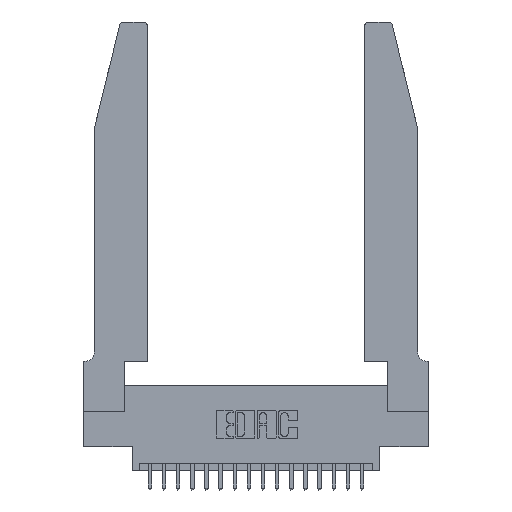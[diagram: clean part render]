
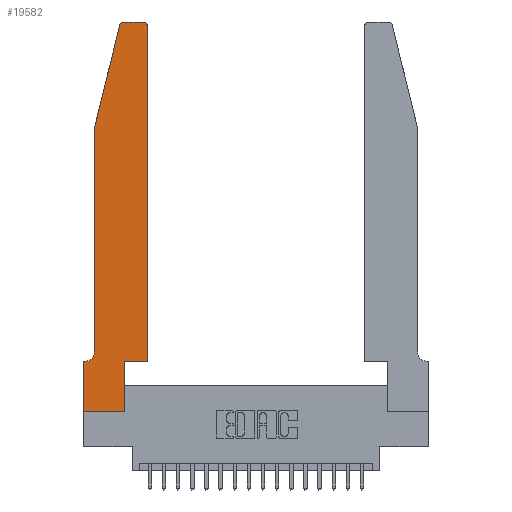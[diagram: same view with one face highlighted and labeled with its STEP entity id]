
A CAD part, top view. The second image highlights one B-rep face of the part: STEP entity #19582.
In plain terms, the highlighted planar face has unit normal (0, 0, 1).
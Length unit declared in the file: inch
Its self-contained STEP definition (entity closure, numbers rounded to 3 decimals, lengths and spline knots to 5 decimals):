
#254 = CARTESIAN_POINT ( 'NONE',  ( 0.284, 2.72, 0.37 ) ) ;
#951 = EDGE_CURVE ( 'NONE', #15937, #16300, #12859, .T. ) ;
#1006 = VECTOR ( 'NONE', #16605, 39.37008 ) ;
#1920 = DIRECTION ( 'NONE',  ( 1., 0., 0. ) ) ;
#2243 = DIRECTION ( 'NONE',  ( 1., 0., 0. ) ) ;
#2263 = DIRECTION ( 'NONE',  ( 0., -1., 0. ) ) ;
#2414 = CARTESIAN_POINT ( 'NONE',  ( 0.4505, 0.35, 0.37 ) ) ;
#2462 = AXIS2_PLACEMENT_3D ( 'NONE', #9219, #19206, #9296 ) ;
#2728 = CARTESIAN_POINT ( 'NONE',  ( 0., 0., 0.37 ) ) ;
#2730 = CIRCLE ( 'NONE', #2462, 0.03 ) ;
#2776 = VECTOR ( 'NONE', #20815, 39.37008 ) ;
#2783 = ORIENTED_EDGE ( 'NONE', *, *, #6001, .T. ) ;
#3015 = EDGE_CURVE ( 'NONE', #16300, #16462, #18865, .T. ) ;
#3296 = ORIENTED_EDGE ( 'NONE', *, *, #18633, .T. ) ;
#3348 = VERTEX_POINT ( 'NONE', #7384 ) ;
#3589 = CARTESIAN_POINT ( 'NONE',  ( 0.4505, 0.35, 0.37 ) ) ;
#3684 = CARTESIAN_POINT ( 'NONE',  ( 0.2605, 2.75, 0.37 ) ) ;
#3708 = EDGE_CURVE ( 'NONE', #10830, #5366, #13779, .T. ) ;
#3913 = CARTESIAN_POINT ( 'NONE',  ( 0.0755, 2., 0.37 ) ) ;
#4229 = DIRECTION ( 'NONE',  ( 0., 0., 1. ) ) ;
#4475 = AXIS2_PLACEMENT_3D ( 'NONE', #20139, #4229, #7178 ) ;
#5235 = ORIENTED_EDGE ( 'NONE', *, *, #12095, .T. ) ;
#5366 = VERTEX_POINT ( 'NONE', #3913 ) ;
#5516 = CARTESIAN_POINT ( 'NONE',  ( 0.4505, 2.72, 0.37 ) ) ;
#6001 = EDGE_CURVE ( 'NONE', #3348, #19127, #7331, .T. ) ;
#6532 = ORIENTED_EDGE ( 'NONE', *, *, #20228, .T. ) ;
#7178 = DIRECTION ( 'NONE',  ( 1., 0., 0. ) ) ;
#7331 = LINE ( 'NONE', #3684, #1006 ) ;
#7384 = CARTESIAN_POINT ( 'NONE',  ( 0.4205, 2.75, 0.37 ) ) ;
#7791 = VERTEX_POINT ( 'NONE', #15082 ) ;
#8254 = VECTOR ( 'NONE', #20653, 39.37008 ) ;
#8448 = ORIENTED_EDGE ( 'NONE', *, *, #3708, .T. ) ;
#8888 = CARTESIAN_POINT ( 'NONE',  ( 0.0755, 2., 0.37 ) ) ;
#8972 = EDGE_CURVE ( 'NONE', #18803, #3348, #2730, .T. ) ;
#8998 = DIRECTION ( 'NONE',  ( -1., 0., 0. ) ) ;
#9218 = EDGE_CURVE ( 'NONE', #12916, #7791, #14391, .T. ) ;
#9219 = CARTESIAN_POINT ( 'NONE',  ( 0.4205, 2.72, 0.37 ) ) ;
#9296 = DIRECTION ( 'NONE',  ( 1., 0., 0. ) ) ;
#9396 = VERTEX_POINT ( 'NONE', #20106 ) ;
#9602 = AXIS2_PLACEMENT_3D ( 'NONE', #254, #11808, #1920 ) ;
#9863 = CARTESIAN_POINT ( 'NONE',  ( 0.2865, 0., 0.37 ) ) ;
#10069 = CARTESIAN_POINT ( 'NONE',  ( 0.2865, 0.35, 0.37 ) ) ;
#10567 = CARTESIAN_POINT ( 'NONE',  ( 0., 0.35, 0.37 ) ) ;
#10830 = VERTEX_POINT ( 'NONE', #19208 ) ;
#10852 = DIRECTION ( 'NONE',  ( 1., 0., 0. ) ) ;
#11147 = LINE ( 'NONE', #3589, #16670 ) ;
#11283 = VECTOR ( 'NONE', #2263, 39.37008 ) ;
#11411 = ORIENTED_EDGE ( 'NONE', *, *, #16134, .T. ) ;
#11548 = DIRECTION ( 'NONE',  ( -1., 0., 0. ) ) ;
#11775 = ORIENTED_EDGE ( 'NONE', *, *, #951, .T. ) ;
#11795 = EDGE_LOOP ( 'NONE', ( #2783, #3296, #8448, #11411, #18312, #17754, #11775, #20125, #6532, #14530, #5235, #15526 ) ) ;
#11808 = DIRECTION ( 'NONE',  ( 0., 0., 1. ) ) ;
#12095 = EDGE_CURVE ( 'NONE', #9396, #18803, #14563, .T. ) ;
#12621 = CARTESIAN_POINT ( 'NONE',  ( 0.2865, 0.35, 0.37 ) ) ;
#12859 = LINE ( 'NONE', #19000, #8254 ) ;
#12916 = VERTEX_POINT ( 'NONE', #15480 ) ;
#13384 = LINE ( 'NONE', #12621, #2776 ) ;
#13591 = AXIS2_PLACEMENT_3D ( 'NONE', #15013, #18112, #11548 ) ;
#13771 = PLANE ( 'NONE',  #4475 ) ;
#13779 = LINE ( 'NONE', #15147, #14807 ) ;
#14391 = CIRCLE ( 'NONE', #13591, 0.07 ) ;
#14530 = ORIENTED_EDGE ( 'NONE', *, *, #19485, .T. ) ;
#14563 = LINE ( 'NONE', #2414, #17798 ) ;
#14612 = VECTOR ( 'NONE', #10852, 39.37008 ) ;
#14807 = VECTOR ( 'NONE', #15284, 39.37008 ) ;
#15013 = CARTESIAN_POINT ( 'NONE',  ( 0.0055, 0.42, 0.37 ) ) ;
#15082 = CARTESIAN_POINT ( 'NONE',  ( 0.0055, 0.35, 0.37 ) ) ;
#15147 = CARTESIAN_POINT ( 'NONE',  ( 0.0755, 2., 0.37 ) ) ;
#15284 = DIRECTION ( 'NONE',  ( -0.239, -0.971, 0. ) ) ;
#15480 = CARTESIAN_POINT ( 'NONE',  ( 0.0755, 0.42, 0.37 ) ) ;
#15526 = ORIENTED_EDGE ( 'NONE', *, *, #8972, .T. ) ;
#15777 = VERTEX_POINT ( 'NONE', #10069 ) ;
#15937 = VERTEX_POINT ( 'NONE', #10567 ) ;
#16134 = EDGE_CURVE ( 'NONE', #5366, #12916, #18640, .T. ) ;
#16300 = VERTEX_POINT ( 'NONE', #19081 ) ;
#16462 = VERTEX_POINT ( 'NONE', #9863 ) ;
#16605 = DIRECTION ( 'NONE',  ( -1., 0., 0. ) ) ;
#16670 = VECTOR ( 'NONE', #2243, 39.37008 ) ;
#17672 = CARTESIAN_POINT ( 'NONE',  ( 0.284, 2.75, 0.37 ) ) ;
#17754 = ORIENTED_EDGE ( 'NONE', *, *, #20199, .T. ) ;
#17798 = VECTOR ( 'NONE', #20172, 39.37008 ) ;
#18112 = DIRECTION ( 'NONE',  ( 0., 0., -1. ) ) ;
#18312 = ORIENTED_EDGE ( 'NONE', *, *, #9218, .T. ) ;
#18435 = VECTOR ( 'NONE', #8998, 39.37008 ) ;
#18633 = EDGE_CURVE ( 'NONE', #19127, #10830, #19014, .T. ) ;
#18640 = LINE ( 'NONE', #8888, #11283 ) ;
#18682 = CARTESIAN_POINT ( 'NONE',  ( 0.0755, 0.35, 0.37 ) ) ;
#18803 = VERTEX_POINT ( 'NONE', #5516 ) ;
#18865 = LINE ( 'NONE', #2728, #14612 ) ;
#19000 = CARTESIAN_POINT ( 'NONE',  ( 0., 0., 0.37 ) ) ;
#19014 = CIRCLE ( 'NONE', #9602, 0.03 ) ;
#19081 = CARTESIAN_POINT ( 'NONE',  ( 0., 0., 0.37 ) ) ;
#19127 = VERTEX_POINT ( 'NONE', #17672 ) ;
#19206 = DIRECTION ( 'NONE',  ( 0., 0., 1. ) ) ;
#19208 = CARTESIAN_POINT ( 'NONE',  ( 0.25487, 2.72718, 0.37 ) ) ;
#19243 = FACE_OUTER_BOUND ( 'NONE', #11795, .T. ) ;
#19485 = EDGE_CURVE ( 'NONE', #15777, #9396, #11147, .T. ) ;
#19582 = ADVANCED_FACE ( 'NONE', ( #19243 ), #13771, .T. ) ;
#20106 = CARTESIAN_POINT ( 'NONE',  ( 0.4505, 0.35, 0.37 ) ) ;
#20125 = ORIENTED_EDGE ( 'NONE', *, *, #3015, .T. ) ;
#20139 = CARTESIAN_POINT ( 'NONE',  ( 0., 0.35, 0.37 ) ) ;
#20172 = DIRECTION ( 'NONE',  ( 0., 1., 0. ) ) ;
#20199 = EDGE_CURVE ( 'NONE', #7791, #15937, #20221, .T. ) ;
#20221 = LINE ( 'NONE', #18682, #18435 ) ;
#20228 = EDGE_CURVE ( 'NONE', #16462, #15777, #13384, .T. ) ;
#20653 = DIRECTION ( 'NONE',  ( 0., -1., 0. ) ) ;
#20815 = DIRECTION ( 'NONE',  ( 0., 1., 0. ) ) ;
